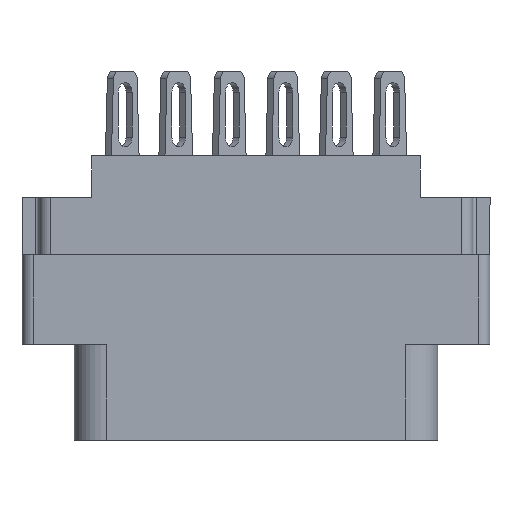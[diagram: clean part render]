
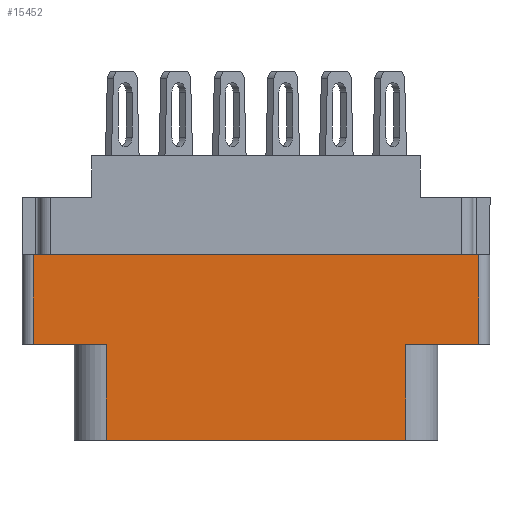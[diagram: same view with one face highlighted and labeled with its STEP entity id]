
A CAD part, front view. The second image highlights one B-rep face of the part: STEP entity #15452.
In plain terms, the highlighted planar face has unit normal (0, -1, 0).
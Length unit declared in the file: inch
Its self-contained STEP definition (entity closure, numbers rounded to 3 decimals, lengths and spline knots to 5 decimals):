
#113 = VERTEX_POINT ( 'NONE', #11952 ) ;
#272 = CARTESIAN_POINT ( 'NONE',  ( -0.624, -0.343, -0.798 ) ) ;
#754 = CARTESIAN_POINT ( 'NONE',  ( 0.42, -0.343, -0.529 ) ) ;
#2100 = VECTOR ( 'NONE', #19158, 39.37008 ) ;
#2250 = EDGE_LOOP ( 'NONE', ( #16491, #7528, #4816, #14547, #5254, #16682, #8958, #13821 ) ) ;
#3212 = EDGE_CURVE ( 'NONE', #12954, #14229, #11117, .T. ) ;
#3414 = VERTEX_POINT ( 'NONE', #15413 ) ;
#3747 = CARTESIAN_POINT ( 'NONE',  ( 0.624, -0.343, -0.798 ) ) ;
#3999 = LINE ( 'NONE', #3747, #2100 ) ;
#4271 = DIRECTION ( 'NONE',  ( 1., 0., 0. ) ) ;
#4555 = VERTEX_POINT ( 'NONE', #14266 ) ;
#4816 = ORIENTED_EDGE ( 'NONE', *, *, #19293, .F. ) ;
#4936 = CARTESIAN_POINT ( 'NONE',  ( 0.624, -0.343, -0.529 ) ) ;
#5143 = CARTESIAN_POINT ( 'NONE',  ( -0.624, -0.343, -0.798 ) ) ;
#5254 = ORIENTED_EDGE ( 'NONE', *, *, #16356, .T. ) ;
#5718 = VECTOR ( 'NONE', #6172, 39.37008 ) ;
#6172 = DIRECTION ( 'NONE',  ( 1., 0., 0. ) ) ;
#6480 = PLANE ( 'NONE',  #15407 ) ;
#6671 = LINE ( 'NONE', #9154, #18950 ) ;
#7260 = VECTOR ( 'NONE', #16094, 39.37008 ) ;
#7528 = ORIENTED_EDGE ( 'NONE', *, *, #13101, .T. ) ;
#7712 = CARTESIAN_POINT ( 'NONE',  ( -0.656, -0.343, -0.277 ) ) ;
#7823 = EDGE_CURVE ( 'NONE', #9211, #4555, #6671, .T. ) ;
#8095 = EDGE_CURVE ( 'NONE', #16985, #12954, #11722, .T. ) ;
#8958 = ORIENTED_EDGE ( 'NONE', *, *, #10720, .F. ) ;
#8965 = CARTESIAN_POINT ( 'NONE',  ( 0., -0.343, -0.529 ) ) ;
#9154 = CARTESIAN_POINT ( 'NONE',  ( 0., -0.343, -0.529 ) ) ;
#9211 = VERTEX_POINT ( 'NONE', #4936 ) ;
#10482 = DIRECTION ( 'NONE',  ( 0., 0., -1. ) ) ;
#10652 = DIRECTION ( 'NONE',  ( -1., 0., 0. ) ) ;
#10720 = EDGE_CURVE ( 'NONE', #16985, #14262, #13528, .T. ) ;
#11011 = DIRECTION ( 'NONE',  ( 0., 0., -1. ) ) ;
#11117 = LINE ( 'NONE', #13300, #11824 ) ;
#11487 = VECTOR ( 'NONE', #14336, 39.37008 ) ;
#11722 = LINE ( 'NONE', #8965, #12436 ) ;
#11824 = VECTOR ( 'NONE', #10482, 39.37008 ) ;
#11952 = CARTESIAN_POINT ( 'NONE',  ( 0.42, -0.343, -0.798 ) ) ;
#12424 = DIRECTION ( 'NONE',  ( 0., -1., 0. ) ) ;
#12436 = VECTOR ( 'NONE', #4271, 39.37008 ) ;
#12718 = FACE_OUTER_BOUND ( 'NONE', #2250, .T. ) ;
#12938 = CARTESIAN_POINT ( 'NONE',  ( -0.624, -0.343, -0.277 ) ) ;
#12954 = VERTEX_POINT ( 'NONE', #14207 ) ;
#13023 = EDGE_CURVE ( 'NONE', #14262, #3414, #16338, .T. ) ;
#13101 = EDGE_CURVE ( 'NONE', #14229, #113, #17531, .T. ) ;
#13300 = CARTESIAN_POINT ( 'NONE',  ( -0.42, -0.343, -0.529 ) ) ;
#13528 = LINE ( 'NONE', #14237, #17400 ) ;
#13821 = ORIENTED_EDGE ( 'NONE', *, *, #8095, .T. ) ;
#14207 = CARTESIAN_POINT ( 'NONE',  ( -0.42, -0.343, -0.529 ) ) ;
#14229 = VERTEX_POINT ( 'NONE', #16182 ) ;
#14237 = CARTESIAN_POINT ( 'NONE',  ( -0.624, -0.343, -0.798 ) ) ;
#14262 = VERTEX_POINT ( 'NONE', #12938 ) ;
#14266 = CARTESIAN_POINT ( 'NONE',  ( 0.42, -0.343, -0.529 ) ) ;
#14336 = DIRECTION ( 'NONE',  ( 1., 0., 0. ) ) ;
#14547 = ORIENTED_EDGE ( 'NONE', *, *, #7823, .F. ) ;
#15407 = AXIS2_PLACEMENT_3D ( 'NONE', #272, #12424, #11011 ) ;
#15413 = CARTESIAN_POINT ( 'NONE',  ( 0.624, -0.343, -0.277 ) ) ;
#15452 = ADVANCED_FACE ( 'NONE', ( #12718 ), #6480, .T. ) ;
#16094 = DIRECTION ( 'NONE',  ( 0., 0., -1. ) ) ;
#16182 = CARTESIAN_POINT ( 'NONE',  ( -0.42, -0.343, -0.798 ) ) ;
#16338 = LINE ( 'NONE', #7712, #5718 ) ;
#16356 = EDGE_CURVE ( 'NONE', #9211, #3414, #3999, .T. ) ;
#16491 = ORIENTED_EDGE ( 'NONE', *, *, #3212, .T. ) ;
#16682 = ORIENTED_EDGE ( 'NONE', *, *, #13023, .F. ) ;
#16985 = VERTEX_POINT ( 'NONE', #17619 ) ;
#17331 = DIRECTION ( 'NONE',  ( 0., 0., 1. ) ) ;
#17400 = VECTOR ( 'NONE', #17331, 39.37008 ) ;
#17531 = LINE ( 'NONE', #5143, #11487 ) ;
#17619 = CARTESIAN_POINT ( 'NONE',  ( -0.624, -0.343, -0.529 ) ) ;
#17643 = LINE ( 'NONE', #754, #7260 ) ;
#18950 = VECTOR ( 'NONE', #10652, 39.37008 ) ;
#19158 = DIRECTION ( 'NONE',  ( 0., 0., 1. ) ) ;
#19293 = EDGE_CURVE ( 'NONE', #4555, #113, #17643, .T. ) ;
